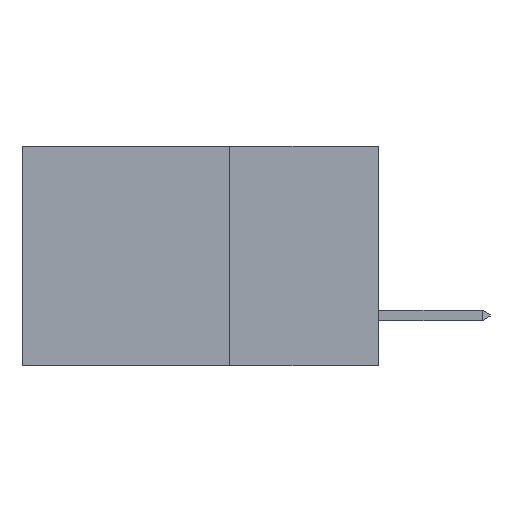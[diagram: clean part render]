
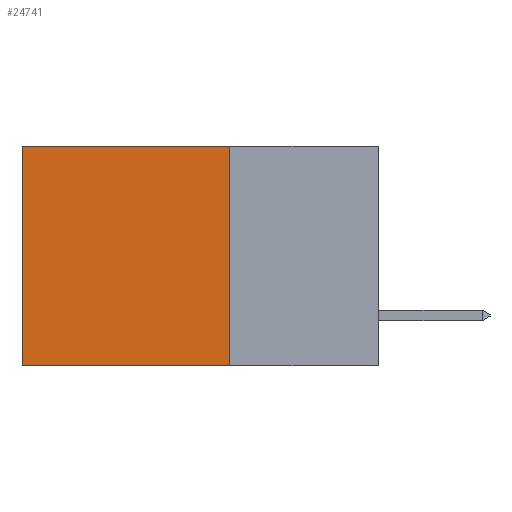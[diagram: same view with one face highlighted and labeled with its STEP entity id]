
A CAD part, left-side view. The second image highlights one B-rep face of the part: STEP entity #24741.
In plain terms, the highlighted planar face has unit normal (-1, 0, 0).
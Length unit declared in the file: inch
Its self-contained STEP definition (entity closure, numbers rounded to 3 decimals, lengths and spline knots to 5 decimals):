
#3094 = EDGE_CURVE ( 'NONE', #3320, #17909, #4044, .T. ) ;
#3320 = VERTEX_POINT ( 'NONE', #12015 ) ;
#4044 = LINE ( 'NONE', #16784, #20370 ) ;
#4455 = CARTESIAN_POINT ( 'NONE',  ( 0.298, 0.6, 0. ) ) ;
#4500 = FACE_OUTER_BOUND ( 'NONE', #22553, .T. ) ;
#4523 = EDGE_CURVE ( 'NONE', #7258, #7286, #15180, .T. ) ;
#4666 = CARTESIAN_POINT ( 'NONE',  ( 0.298, 0.25, 0. ) ) ;
#4860 = CARTESIAN_POINT ( 'NONE',  ( 0.298, 0.6, -0.37 ) ) ;
#5072 = ORIENTED_EDGE ( 'NONE', *, *, #18594, .T. ) ;
#5453 = CARTESIAN_POINT ( 'NONE',  ( 0.298, 0.25, 0. ) ) ;
#6811 = ORIENTED_EDGE ( 'NONE', *, *, #19868, .F. ) ;
#7258 = VERTEX_POINT ( 'NONE', #5453 ) ;
#7286 = VERTEX_POINT ( 'NONE', #4455 ) ;
#8121 = DIRECTION ( 'NONE',  ( 1., 0., 0. ) ) ;
#9973 = LINE ( 'NONE', #20964, #25478 ) ;
#10483 = DIRECTION ( 'NONE',  ( 0., 0., -1. ) ) ;
#12015 = CARTESIAN_POINT ( 'NONE',  ( 0.298, 0.25, -0.37 ) ) ;
#15180 = LINE ( 'NONE', #4666, #25274 ) ;
#15350 = LINE ( 'NONE', #18808, #20767 ) ;
#15761 = AXIS2_PLACEMENT_3D ( 'NONE', #20251, #8121, #22363 ) ;
#16695 = DIRECTION ( 'NONE',  ( 0., 1., 0. ) ) ;
#16784 = CARTESIAN_POINT ( 'NONE',  ( 0.298, 0.25, -0.37 ) ) ;
#17909 = VERTEX_POINT ( 'NONE', #4860 ) ;
#18063 = DIRECTION ( 'NONE',  ( 0., 1., 0. ) ) ;
#18594 = EDGE_CURVE ( 'NONE', #7286, #17909, #9973, .T. ) ;
#18808 = CARTESIAN_POINT ( 'NONE',  ( 0.298, 0.25, 0. ) ) ;
#19609 = ORIENTED_EDGE ( 'NONE', *, *, #3094, .F. ) ;
#19868 = EDGE_CURVE ( 'NONE', #7258, #3320, #15350, .T. ) ;
#20251 = CARTESIAN_POINT ( 'NONE',  ( 0.298, 0.25, 0. ) ) ;
#20332 = PLANE ( 'NONE',  #15761 ) ;
#20370 = VECTOR ( 'NONE', #16695, 39.37008 ) ;
#20767 = VECTOR ( 'NONE', #10483, 39.37008 ) ;
#20964 = CARTESIAN_POINT ( 'NONE',  ( 0.298, 0.6, 0. ) ) ;
#22363 = DIRECTION ( 'NONE',  ( 0., 0., -1. ) ) ;
#22553 = EDGE_LOOP ( 'NONE', ( #5072, #19609, #6811, #25240 ) ) ;
#23001 = DIRECTION ( 'NONE',  ( 0., 0., -1. ) ) ;
#24741 = ADVANCED_FACE ( 'NONE', ( #4500 ), #20332, .F. ) ;
#25240 = ORIENTED_EDGE ( 'NONE', *, *, #4523, .T. ) ;
#25274 = VECTOR ( 'NONE', #18063, 39.37008 ) ;
#25478 = VECTOR ( 'NONE', #23001, 39.37008 ) ;
